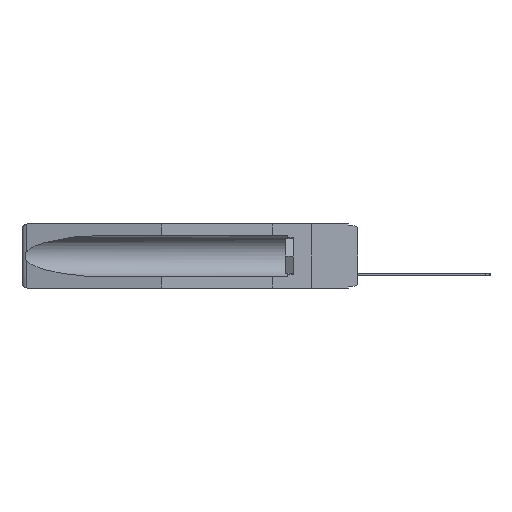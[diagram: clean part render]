
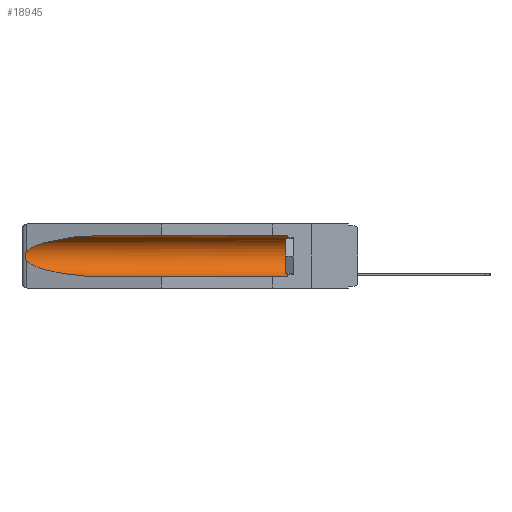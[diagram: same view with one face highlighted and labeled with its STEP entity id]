
A CAD part, left-side view. The second image highlights one B-rep face of the part: STEP entity #18945.
In plain terms, the highlighted cylindrical face has radius 2.857 mm (diameter 5.715 mm), a partial arc.
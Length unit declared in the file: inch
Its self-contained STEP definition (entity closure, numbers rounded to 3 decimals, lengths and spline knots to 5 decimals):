
#368 = CARTESIAN_POINT ( 'NONE',  ( 0.155, -0.30754, -0.059 ) ) ;
#424 = CARTESIAN_POINT ( 'NONE',  ( 0.2673, 1.53269, -0.17917 ) ) ;
#483 = CARTESIAN_POINT ( 'NONE',  ( 0.25451, 1.48313, -0.24835 ) ) ;
#790 = CARTESIAN_POINT ( 'NONE',  ( 0.26537, 1.52718, -0.19328 ) ) ;
#934 = CARTESIAN_POINT ( 'NONE',  ( 0.21114, 1.30732, -0.059 ) ) ;
#1205 = AXIS2_PLACEMENT_3D ( 'NONE', #8851, #16169, #23500 ) ;
#1518 = CYLINDRICAL_SURFACE ( 'NONE', #1205, 0.1125 ) ;
#2296 = CARTESIAN_POINT ( 'NONE',  ( 0.26537, 1.52718, -0.19328 ) ) ;
#2423 = LINE ( 'NONE', #368, #13375 ) ;
#2446 = EDGE_LOOP ( 'NONE', ( #18579, #22662, #6770, #14344, #20392, #2538 ) ) ;
#2538 = ORIENTED_EDGE ( 'NONE', *, *, #16417, .T. ) ;
#2751 = EDGE_CURVE ( 'NONE', #15105, #8692, #11773, .T. ) ;
#2887 = CARTESIAN_POINT ( 'NONE',  ( 0.155, -0.30754, -0.284 ) ) ;
#3914 = CARTESIAN_POINT ( 'NONE',  ( 0.26537, 1.52718, -0.14972 ) ) ;
#4077 = CARTESIAN_POINT ( 'NONE',  ( 0.26537, 1.52718, -0.14972 ) ) ;
#4413 = CARTESIAN_POINT ( 'NONE',  ( 0.26537, 1.52718, -0.14972 ) ) ;
#5418 = AXIS2_PLACEMENT_3D ( 'NONE', #21818, #14246, #8970 ) ;
#5481 = EDGE_CURVE ( 'NONE', #20052, #18962, #13624, .T. ) ;
#5669 = CARTESIAN_POINT ( 'NONE',  ( 0.155, 1.07973, -0.284 ) ) ;
#5852 = CARTESIAN_POINT ( 'NONE',  ( 0.26654, 1.53092, -0.15636 ) ) ;
#6770 = ORIENTED_EDGE ( 'NONE', *, *, #22382, .T. ) ;
#7776 = VERTEX_POINT ( 'NONE', #19004 ) ;
#7895 = CARTESIAN_POINT ( 'NONE',  ( 0.2675, 1.53308, -0.16763 ) ) ;
#8155 = CARTESIAN_POINT ( 'NONE',  ( 0.25451, 1.48313, -0.09465 ) ) ;
#8267 = CARTESIAN_POINT ( 'NONE',  ( 0.155, 1.07973, -0.059 ) ) ;
#8692 = VERTEX_POINT ( 'NONE', #11847 ) ;
#8851 = CARTESIAN_POINT ( 'NONE',  ( 0.155, -0.30754, -0.1715 ) ) ;
#8970 = DIRECTION ( 'NONE',  ( 0., 0., 1. ) ) ;
#9497 =( BOUNDED_CURVE ( )  B_SPLINE_CURVE ( 3, ( #2296, #483, #20550, #5669 ),
 .UNSPECIFIED., .F., .F. ) 
 B_SPLINE_CURVE_WITH_KNOTS ( ( 4, 4 ),
 ( 0.1948, 1.5708 ),
 .UNSPECIFIED. ) 
 CURVE ( )  GEOMETRIC_REPRESENTATION_ITEM ( )  RATIONAL_B_SPLINE_CURVE ( ( 1., 0.848, 0.848, 1. ) ) 
 REPRESENTATION_ITEM ( '' )  );
#10655 = FACE_OUTER_BOUND ( 'NONE', #2446, .T. ) ;
#11604 = CARTESIAN_POINT ( 'NONE',  ( 0.26655, 1.53094, -0.18657 ) ) ;
#11773 = LINE ( 'NONE', #2887, #21006 ) ;
#11847 = CARTESIAN_POINT ( 'NONE',  ( 0.155, 1.07973, -0.284 ) ) ;
#12936 = EDGE_CURVE ( 'NONE', #18962, #15028, #14340, .T. ) ;
#13167 = CARTESIAN_POINT ( 'NONE',  ( 0.2673, 1.5327, -0.16383 ) ) ;
#13375 = VECTOR ( 'NONE', #20676, 39.37008 ) ;
#13427 = CARTESIAN_POINT ( 'NONE',  ( 0.155, 1.07973, -0.059 ) ) ;
#13624 =( BOUNDED_CURVE ( )  B_SPLINE_CURVE ( 3, ( #13427, #934, #8155, #4077 ),
 .UNSPECIFIED., .F., .F. ) 
 B_SPLINE_CURVE_WITH_KNOTS ( ( 4, 4 ),
 ( 4.71239, 6.08839 ),
 .UNSPECIFIED. ) 
 CURVE ( )  GEOMETRIC_REPRESENTATION_ITEM ( )  RATIONAL_B_SPLINE_CURVE ( ( 1., 0.848, 0.848, 1. ) ) 
 REPRESENTATION_ITEM ( '' )  );
#14246 = DIRECTION ( 'NONE',  ( 0., -1., 0. ) ) ;
#14340 = B_SPLINE_CURVE_WITH_KNOTS ( 'NONE', 3,
 ( #4413, #22302, #5852, #13167, #7895, #20497, #424, #11604, #17016, #790 ),
 .UNSPECIFIED., .F., .F.,
 ( 4, 2, 2, 2, 4 ),
 ( 0., 0.00029, 0.00058, 0.00087, 0.00117 ),
 .UNSPECIFIED. ) ;
#14344 = ORIENTED_EDGE ( 'NONE', *, *, #2751, .F. ) ;
#15028 = VERTEX_POINT ( 'NONE', #16612 ) ;
#15105 = VERTEX_POINT ( 'NONE', #22020 ) ;
#15243 = DIRECTION ( 'NONE',  ( 0., 1., 0. ) ) ;
#16169 = DIRECTION ( 'NONE',  ( 0., 1., 0. ) ) ;
#16417 = EDGE_CURVE ( 'NONE', #7776, #20052, #2423, .T. ) ;
#16612 = CARTESIAN_POINT ( 'NONE',  ( 0.26537, 1.52718, -0.19328 ) ) ;
#17016 = CARTESIAN_POINT ( 'NONE',  ( 0.26597, 1.5296, -0.19026 ) ) ;
#17713 = CIRCLE ( 'NONE', #5418, 0.1125 ) ;
#18579 = ORIENTED_EDGE ( 'NONE', *, *, #5481, .T. ) ;
#18856 = EDGE_CURVE ( 'NONE', #15105, #7776, #17713, .T. ) ;
#18945 = ADVANCED_FACE ( 'NONE', ( #10655 ), #1518, .F. ) ;
#18962 = VERTEX_POINT ( 'NONE', #3914 ) ;
#19004 = CARTESIAN_POINT ( 'NONE',  ( 0.155, 0.126, -0.059 ) ) ;
#20052 = VERTEX_POINT ( 'NONE', #8267 ) ;
#20392 = ORIENTED_EDGE ( 'NONE', *, *, #18856, .T. ) ;
#20497 = CARTESIAN_POINT ( 'NONE',  ( 0.2675, 1.53308, -0.17534 ) ) ;
#20550 = CARTESIAN_POINT ( 'NONE',  ( 0.21114, 1.30732, -0.284 ) ) ;
#20676 = DIRECTION ( 'NONE',  ( 0., 1., 0. ) ) ;
#21006 = VECTOR ( 'NONE', #15243, 39.37008 ) ;
#21818 = CARTESIAN_POINT ( 'NONE',  ( 0.155, 0.126, -0.1715 ) ) ;
#22020 = CARTESIAN_POINT ( 'NONE',  ( 0.155, 0.126, -0.284 ) ) ;
#22302 = CARTESIAN_POINT ( 'NONE',  ( 0.26597, 1.52961, -0.15275 ) ) ;
#22382 = EDGE_CURVE ( 'NONE', #15028, #8692, #9497, .T. ) ;
#22662 = ORIENTED_EDGE ( 'NONE', *, *, #12936, .T. ) ;
#23500 = DIRECTION ( 'NONE',  ( 0., 0., 1. ) ) ;
